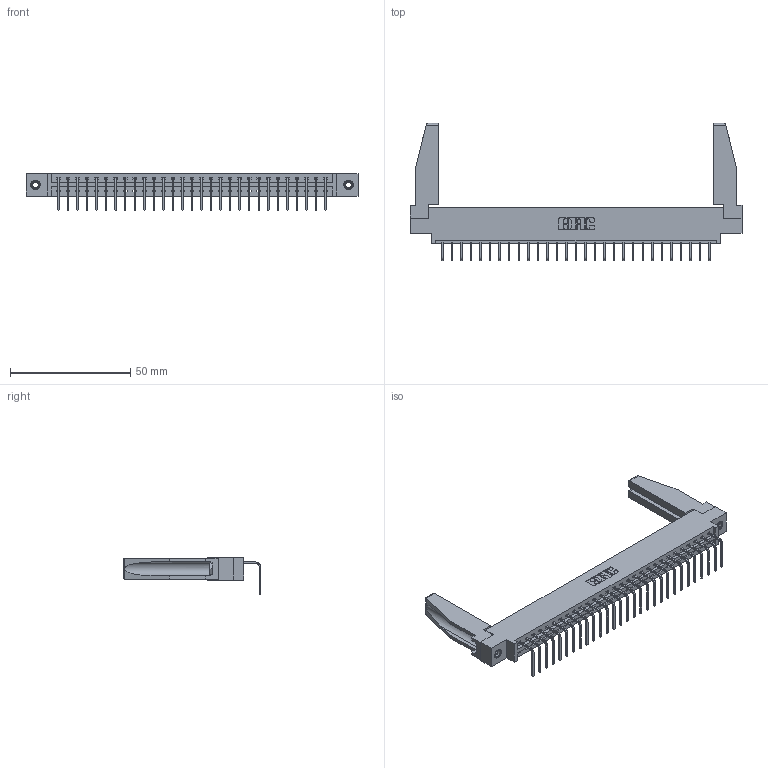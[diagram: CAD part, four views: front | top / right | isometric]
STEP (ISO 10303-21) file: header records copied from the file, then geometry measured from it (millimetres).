
FILE_DESCRIPTION (( 'STEP AP203' ), '1' );
FILE_NAME ('337-029-558-678.STEP', '2019-10-07T13:38:18', ( '' ), ( '' ), 'SwSTEP 2.0', 'SolidWorks 2016', '' );
FILE_SCHEMA (( 'CONFIG_CONTROL_DESIGN' ));
Length unit declared in the file: inch
Products named in the file (5): 345-292-001_558 Tail - 2; 307-220-078; 337-029-558-678; 345-250-001_345-250-001-102; 337 Part_0.170 Offset - 0.156 Dia-TI
Assembly tree (34 placements, depth 2):
  337-029-558-678
    337 Part_0.170 Offset - 0.156 Dia-TI
    345-292-001_558 Tail - 2  x29
    345-250-001_345-250-001-102  x2
    307-220-078  x2
Bounding box: 137.92 x 56.96 x 15.37 mm (x, y, z)
Volume: 18144.4 mm3; surface area: 19077.8 mm2
Topology: 34 solids, 34 shells, 2104 faces, 6279 edges, 4138 vertices
Faces by surface type: plane 1550, cylinder 538, cone 12, torus 4
Entity records: 25894 total; most frequent: CARTESIAN_POINT 4503, ORIENTED_EDGE 4424, DIRECTION 3826, EDGE_CURVE 2212, LINE 2046, VECTOR 2046, VERTEX_POINT 1468, AXIS2_PLACEMENT_3D 890
